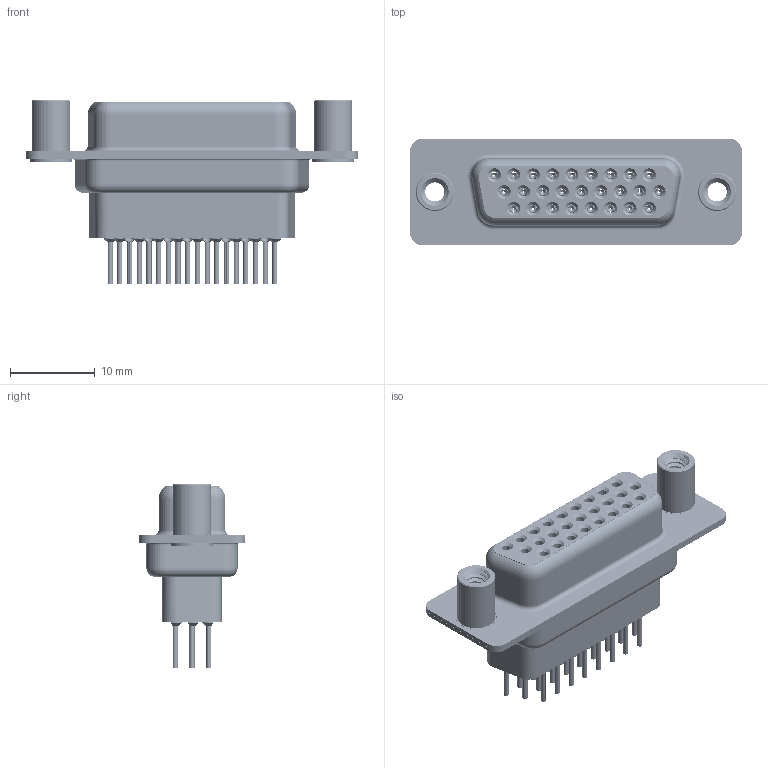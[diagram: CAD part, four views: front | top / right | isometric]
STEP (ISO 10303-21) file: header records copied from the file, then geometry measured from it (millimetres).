
FILE_DESCRIPTION (( 'STEP AP203' ), '1' );
FILE_NAME ('638-026-631-058.STEP', '2020-07-18T21:28:27', ( '' ), ( '' ), 'SwSTEP 2.0', 'SolidWorks 2020', '' );
FILE_SCHEMA (( 'CONFIG_CONTROL_DESIGN' ));
Length unit declared in the file: millimetre
Products named in the file (8): 638 Contact Row 3_31; 638 Housing_26 Contacts HP; 638 Shell Front_26 Contacts; 638 4-40 Threaded Standoff; 638 Shell Rear_26 Contacts; 638 Contact Row 1_31; 638-026-631-058; 638 Contact Row 2_31
Assembly tree (31 placements, depth 2):
  638-026-631-058
    638 Housing_26 Contacts HP
    638 Shell Front_26 Contacts
    638 Shell Rear_26 Contacts
    638 Contact Row 1_31  x9
    638 Contact Row 2_31  x9
    638 Contact Row 3_31  x8
    638 4-40 Threaded Standoff  x2
Bounding box: 39.19 x 12.6 x 21.7 mm (x, y, z)
Volume: 2739.4 mm3; surface area: 10065.7 mm2
Topology: 31 solids, 31 shells, 3511 faces, 8993 edges, 5609 vertices
Faces by surface type: cylinder 1023, plane 875, torus 681, bspline 526, cone 406
Entity records: 33364 total; most frequent: CARTESIAN_POINT 10103, DIRECTION 4716, ORIENTED_EDGE 4478, EDGE_CURVE 2239, AXIS2_PLACEMENT_3D 1967, VERTEX_POINT 1410, EDGE_LOOP 1085, CIRCLE 1065
